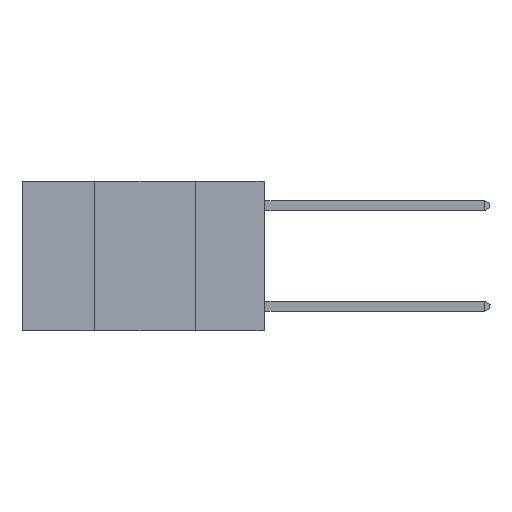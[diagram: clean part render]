
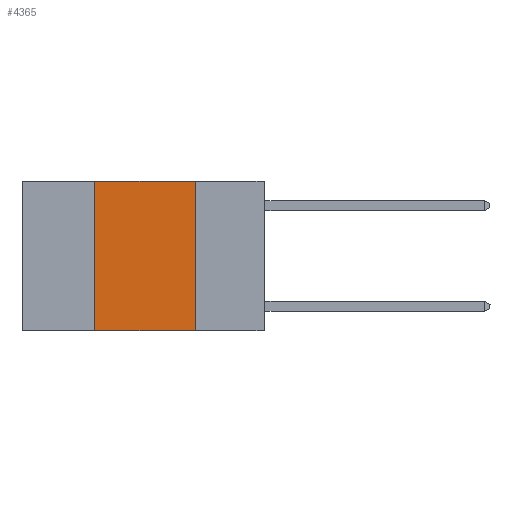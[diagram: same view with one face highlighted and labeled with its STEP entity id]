
A CAD part, left-side view. The second image highlights one B-rep face of the part: STEP entity #4365.
In plain terms, the highlighted planar face has unit normal (-1, 0, 0).
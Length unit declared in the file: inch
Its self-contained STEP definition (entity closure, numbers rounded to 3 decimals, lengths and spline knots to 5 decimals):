
#379 = DIRECTION ( 'NONE',  ( 0., -1., 0. ) ) ;
#826 = VERTEX_POINT ( 'NONE', #4079 ) ;
#1380 = CARTESIAN_POINT ( 'NONE',  ( 0., 0.42, -0.37 ) ) ;
#1491 = CARTESIAN_POINT ( 'NONE',  ( 0., 0.6, 0. ) ) ;
#1822 = EDGE_CURVE ( 'NONE', #1880, #8524, #9097, .T. ) ;
#1851 = CARTESIAN_POINT ( 'NONE',  ( 0., 0.17, 0. ) ) ;
#1880 = VERTEX_POINT ( 'NONE', #1380 ) ;
#2245 = FACE_OUTER_BOUND ( 'NONE', #10117, .T. ) ;
#2524 = DIRECTION ( 'NONE',  ( 0., 0., 1. ) ) ;
#3249 = VECTOR ( 'NONE', #2524, 39.37008 ) ;
#3382 = CARTESIAN_POINT ( 'NONE',  ( 0., 0.17, 0. ) ) ;
#3783 = DIRECTION ( 'NONE',  ( 0., -1., 0. ) ) ;
#4079 = CARTESIAN_POINT ( 'NONE',  ( 0., 0.42, 0. ) ) ;
#4365 = ADVANCED_FACE ( 'NONE', ( #2245 ), #10322, .F. ) ;
#4683 = LINE ( 'NONE', #9726, #4995 ) ;
#4814 = VERTEX_POINT ( 'NONE', #3382 ) ;
#4995 = VECTOR ( 'NONE', #3783, 39.37008 ) ;
#5154 = ORIENTED_EDGE ( 'NONE', *, *, #9321, .F. ) ;
#5642 = AXIS2_PLACEMENT_3D ( 'NONE', #1491, #6964, #9589 ) ;
#6964 = DIRECTION ( 'NONE',  ( 1., 0., 0. ) ) ;
#6972 = EDGE_CURVE ( 'NONE', #826, #4814, #4683, .T. ) ;
#7264 = CARTESIAN_POINT ( 'NONE',  ( 0., 0.6, -0.37 ) ) ;
#8506 = CARTESIAN_POINT ( 'NONE',  ( 0., 0.42, 0. ) ) ;
#8524 = VERTEX_POINT ( 'NONE', #10686 ) ;
#8556 = LINE ( 'NONE', #8506, #3249 ) ;
#8709 = VECTOR ( 'NONE', #10638, 39.37008 ) ;
#9013 = LINE ( 'NONE', #1851, #8709 ) ;
#9097 = LINE ( 'NONE', #7264, #11009 ) ;
#9300 = ORIENTED_EDGE ( 'NONE', *, *, #1822, .T. ) ;
#9321 = EDGE_CURVE ( 'NONE', #4814, #8524, #9013, .T. ) ;
#9589 = DIRECTION ( 'NONE',  ( 0., 0., -1. ) ) ;
#9726 = CARTESIAN_POINT ( 'NONE',  ( 0., 0.6, 0. ) ) ;
#9787 = ORIENTED_EDGE ( 'NONE', *, *, #6972, .F. ) ;
#10117 = EDGE_LOOP ( 'NONE', ( #5154, #9787, #12255, #9300 ) ) ;
#10322 = PLANE ( 'NONE',  #5642 ) ;
#10638 = DIRECTION ( 'NONE',  ( 0., 0., -1. ) ) ;
#10686 = CARTESIAN_POINT ( 'NONE',  ( 0., 0.17, -0.37 ) ) ;
#11009 = VECTOR ( 'NONE', #379, 39.37008 ) ;
#12255 = ORIENTED_EDGE ( 'NONE', *, *, #12446, .F. ) ;
#12446 = EDGE_CURVE ( 'NONE', #1880, #826, #8556, .T. ) ;
